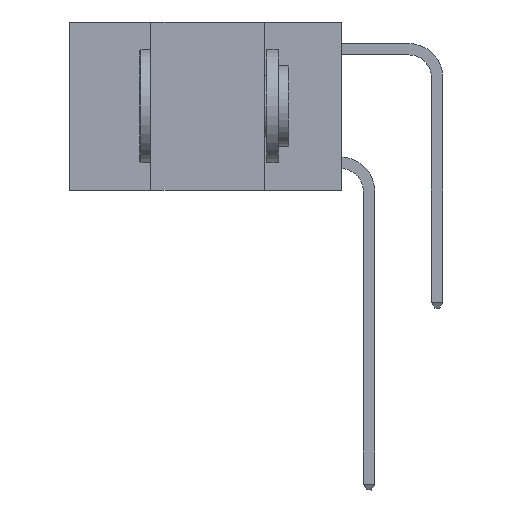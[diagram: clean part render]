
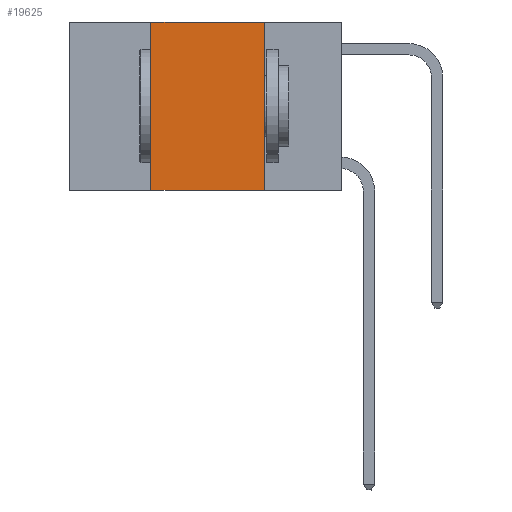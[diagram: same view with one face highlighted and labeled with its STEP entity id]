
A CAD part, left-side view. The second image highlights one B-rep face of the part: STEP entity #19625.
In plain terms, the highlighted planar face has unit normal (-1, 0, 0).
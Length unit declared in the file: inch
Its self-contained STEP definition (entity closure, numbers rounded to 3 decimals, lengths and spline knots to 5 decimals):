
#1743 = LINE ( 'NONE', #13814, #11990 ) ;
#2760 = VECTOR ( 'NONE', #21840, 39.37008 ) ;
#3126 = DIRECTION ( 'NONE',  ( 0., -1., 0. ) ) ;
#3653 = VERTEX_POINT ( 'NONE', #23788 ) ;
#4292 = DIRECTION ( 'NONE',  ( 1., 0., 0. ) ) ;
#4318 = ORIENTED_EDGE ( 'NONE', *, *, #11294, .F. ) ;
#5123 = CARTESIAN_POINT ( 'NONE',  ( 0., 0.42, 0. ) ) ;
#5727 = DIRECTION ( 'NONE',  ( 0., 0., -1. ) ) ;
#8372 = LINE ( 'NONE', #23369, #13141 ) ;
#9452 = FACE_OUTER_BOUND ( 'NONE', #22914, .T. ) ;
#9504 = LINE ( 'NONE', #15732, #2760 ) ;
#9645 = CARTESIAN_POINT ( 'NONE',  ( 0., 0.42, 0. ) ) ;
#10612 = VERTEX_POINT ( 'NONE', #23316 ) ;
#11294 = EDGE_CURVE ( 'NONE', #19217, #21609, #8372, .T. ) ;
#11684 = ORIENTED_EDGE ( 'NONE', *, *, #20104, .F. ) ;
#11990 = VECTOR ( 'NONE', #5727, 39.37008 ) ;
#12410 = PLANE ( 'NONE',  #17768 ) ;
#12623 = ORIENTED_EDGE ( 'NONE', *, *, #25514, .F. ) ;
#13141 = VECTOR ( 'NONE', #3126, 39.37008 ) ;
#13814 = CARTESIAN_POINT ( 'NONE',  ( 0., 0.17, 0. ) ) ;
#15732 = CARTESIAN_POINT ( 'NONE',  ( 0., 0.6, -0.37 ) ) ;
#15757 = DIRECTION ( 'NONE',  ( 0., 0., 1. ) ) ;
#17073 = ORIENTED_EDGE ( 'NONE', *, *, #18738, .T. ) ;
#17483 = CARTESIAN_POINT ( 'NONE',  ( 0., 0.17, 0. ) ) ;
#17768 = AXIS2_PLACEMENT_3D ( 'NONE', #20458, #4292, #18512 ) ;
#18512 = DIRECTION ( 'NONE',  ( 0., 0., -1. ) ) ;
#18738 = EDGE_CURVE ( 'NONE', #10612, #3653, #9504, .T. ) ;
#19217 = VERTEX_POINT ( 'NONE', #5123 ) ;
#19537 = VECTOR ( 'NONE', #15757, 39.37008 ) ;
#19625 = ADVANCED_FACE ( 'NONE', ( #9452 ), #12410, .F. ) ;
#20104 = EDGE_CURVE ( 'NONE', #10612, #19217, #20191, .T. ) ;
#20191 = LINE ( 'NONE', #9645, #19537 ) ;
#20458 = CARTESIAN_POINT ( 'NONE',  ( 0., 0.6, 0. ) ) ;
#21609 = VERTEX_POINT ( 'NONE', #17483 ) ;
#21840 = DIRECTION ( 'NONE',  ( 0., -1., 0. ) ) ;
#22914 = EDGE_LOOP ( 'NONE', ( #12623, #4318, #11684, #17073 ) ) ;
#23316 = CARTESIAN_POINT ( 'NONE',  ( 0., 0.42, -0.37 ) ) ;
#23369 = CARTESIAN_POINT ( 'NONE',  ( 0., 0.6, 0. ) ) ;
#23788 = CARTESIAN_POINT ( 'NONE',  ( 0., 0.17, -0.37 ) ) ;
#25514 = EDGE_CURVE ( 'NONE', #21609, #3653, #1743, .T. ) ;
